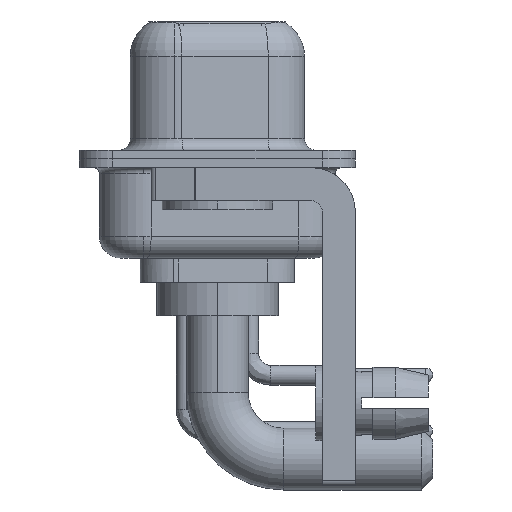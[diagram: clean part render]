
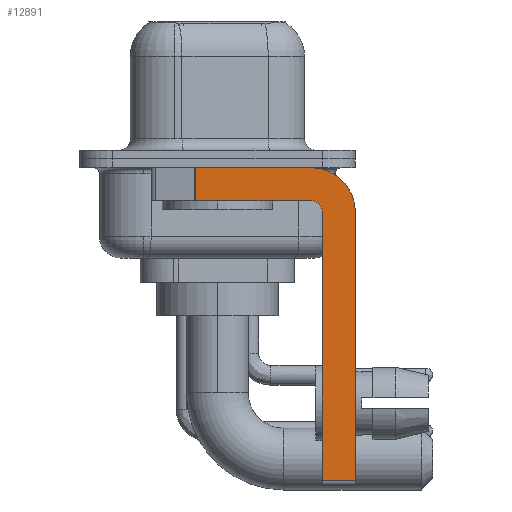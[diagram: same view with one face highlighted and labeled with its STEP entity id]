
A CAD part, left-side view. The second image highlights one B-rep face of the part: STEP entity #12891.
In plain terms, the highlighted planar face has unit normal (-1, 0, 0).
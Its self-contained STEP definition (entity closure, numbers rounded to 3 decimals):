
#65 = LINE ( 'NONE', #11977, #9049 ) ;
#286 = DIRECTION ( 'NONE',  ( 0., 0., -1. ) ) ;
#534 = CARTESIAN_POINT ( 'NONE',  ( -2.9, -6.25, -14.55 ) ) ;
#1107 = CARTESIAN_POINT ( 'NONE',  ( -2.9, -4.75, -2.4 ) ) ;
#1247 = VERTEX_POINT ( 'NONE', #7294 ) ;
#1282 = LINE ( 'NONE', #17484, #10875 ) ;
#1847 = LINE ( 'NONE', #8017, #15471 ) ;
#1989 = CARTESIAN_POINT ( 'NONE',  ( -2.9, -4.25, -14.55 ) ) ;
#2327 = LINE ( 'NONE', #18605, #16012 ) ;
#2416 = ORIENTED_EDGE ( 'NONE', *, *, #14970, .F. ) ;
#2676 = ORIENTED_EDGE ( 'NONE', *, *, #8068, .F. ) ;
#2765 = EDGE_CURVE ( 'NONE', #7150, #1247, #1282, .T. ) ;
#2776 = ORIENTED_EDGE ( 'NONE', *, *, #4502, .F. ) ;
#2962 = DIRECTION ( 'NONE',  ( 0., -1., 0. ) ) ;
#3358 = PLANE ( 'NONE',  #3648 ) ;
#3450 = FACE_OUTER_BOUND ( 'NONE', #4425, .T. ) ;
#3648 = AXIS2_PLACEMENT_3D ( 'NONE', #13788, #9412, #15256 ) ;
#4099 = DIRECTION ( 'NONE',  ( 0., 0., 1. ) ) ;
#4338 = EDGE_CURVE ( 'NONE', #13203, #9324, #13909, .T. ) ;
#4425 = EDGE_LOOP ( 'NONE', ( #7337, #14642, #2776, #15227, #2676, #14281, #2416, #10002 ) ) ;
#4502 = EDGE_CURVE ( 'NONE', #17029, #18187, #7275, .T. ) ;
#4553 = DIRECTION ( 'NONE',  ( 0., 0., -1. ) ) ;
#6478 = CARTESIAN_POINT ( 'NONE',  ( -2.9, -4.25, -2.4 ) ) ;
#7150 = VERTEX_POINT ( 'NONE', #8550 ) ;
#7275 = LINE ( 'NONE', #8743, #18820 ) ;
#7294 = CARTESIAN_POINT ( 'NONE',  ( -2.9, -4.25, -0.4 ) ) ;
#7337 = ORIENTED_EDGE ( 'NONE', *, *, #2765, .F. ) ;
#7390 = EDGE_CURVE ( 'NONE', #1247, #12500, #16618, .T. ) ;
#7811 = CARTESIAN_POINT ( 'NONE',  ( -2.9, -4.25, -1.9 ) ) ;
#8017 = CARTESIAN_POINT ( 'NONE',  ( -2.9, 0.978, -1.9 ) ) ;
#8068 = EDGE_CURVE ( 'NONE', #13203, #8449, #2327, .T. ) ;
#8137 = DIRECTION ( 'NONE',  ( 0., 0., -1. ) ) ;
#8449 = VERTEX_POINT ( 'NONE', #1107 ) ;
#8550 = CARTESIAN_POINT ( 'NONE',  ( -2.9, 0.978, -0.4 ) ) ;
#8743 = CARTESIAN_POINT ( 'NONE',  ( -2.9, -4.25, -1.9 ) ) ;
#8784 = EDGE_CURVE ( 'NONE', #8449, #17029, #17892, .T. ) ;
#9049 = VECTOR ( 'NONE', #4553, 1000. ) ;
#9324 = VERTEX_POINT ( 'NONE', #534 ) ;
#9412 = DIRECTION ( 'NONE',  ( 1., 0., 0. ) ) ;
#9700 = DIRECTION ( 'NONE',  ( -1., 0., 0. ) ) ;
#10002 = ORIENTED_EDGE ( 'NONE', *, *, #7390, .F. ) ;
#10874 = EDGE_CURVE ( 'NONE', #7150, #18187, #1847, .T. ) ;
#10875 = VECTOR ( 'NONE', #2962, 1000. ) ;
#10987 = DIRECTION ( 'NONE',  ( 1., 0., 0. ) ) ;
#11175 = CARTESIAN_POINT ( 'NONE',  ( -2.9, -4.25, -2.4 ) ) ;
#11977 = CARTESIAN_POINT ( 'NONE',  ( -2.9, -6.25, -2.4 ) ) ;
#12260 = AXIS2_PLACEMENT_3D ( 'NONE', #11175, #10987, #8137 ) ;
#12500 = VERTEX_POINT ( 'NONE', #14288 ) ;
#12808 = CARTESIAN_POINT ( 'NONE',  ( -2.9, 0.978, -1.9 ) ) ;
#12891 = ADVANCED_FACE ( 'NONE', ( #3450 ), #3358, .F. ) ;
#13203 = VERTEX_POINT ( 'NONE', #16014 ) ;
#13788 = CARTESIAN_POINT ( 'NONE',  ( -2.9, -4.25, -2.4 ) ) ;
#13792 = DIRECTION ( 'NONE',  ( 0., 0., 1. ) ) ;
#13909 = LINE ( 'NONE', #1989, #15701 ) ;
#14281 = ORIENTED_EDGE ( 'NONE', *, *, #4338, .T. ) ;
#14288 = CARTESIAN_POINT ( 'NONE',  ( -2.9, -6.25, -2.4 ) ) ;
#14642 = ORIENTED_EDGE ( 'NONE', *, *, #10874, .T. ) ;
#14970 = EDGE_CURVE ( 'NONE', #12500, #9324, #65, .T. ) ;
#15227 = ORIENTED_EDGE ( 'NONE', *, *, #8784, .F. ) ;
#15256 = DIRECTION ( 'NONE',  ( 0., 0., -1. ) ) ;
#15471 = VECTOR ( 'NONE', #286, 1000. ) ;
#15643 = DIRECTION ( 'NONE',  ( 0., -1., 0. ) ) ;
#15701 = VECTOR ( 'NONE', #15643, 1000. ) ;
#15937 = DIRECTION ( 'NONE',  ( 0., 1., 0. ) ) ;
#16012 = VECTOR ( 'NONE', #4099, 1000. ) ;
#16014 = CARTESIAN_POINT ( 'NONE',  ( -2.9, -4.75, -14.55 ) ) ;
#16618 = CIRCLE ( 'NONE', #12260, 2. ) ;
#17029 = VERTEX_POINT ( 'NONE', #7811 ) ;
#17276 = AXIS2_PLACEMENT_3D ( 'NONE', #6478, #9700, #13792 ) ;
#17484 = CARTESIAN_POINT ( 'NONE',  ( -2.9, 3., -0.4 ) ) ;
#17892 = CIRCLE ( 'NONE', #17276, 0.5 ) ;
#18187 = VERTEX_POINT ( 'NONE', #12808 ) ;
#18605 = CARTESIAN_POINT ( 'NONE',  ( -2.9, -4.75, -14.8 ) ) ;
#18820 = VECTOR ( 'NONE', #15937, 1000. ) ;
